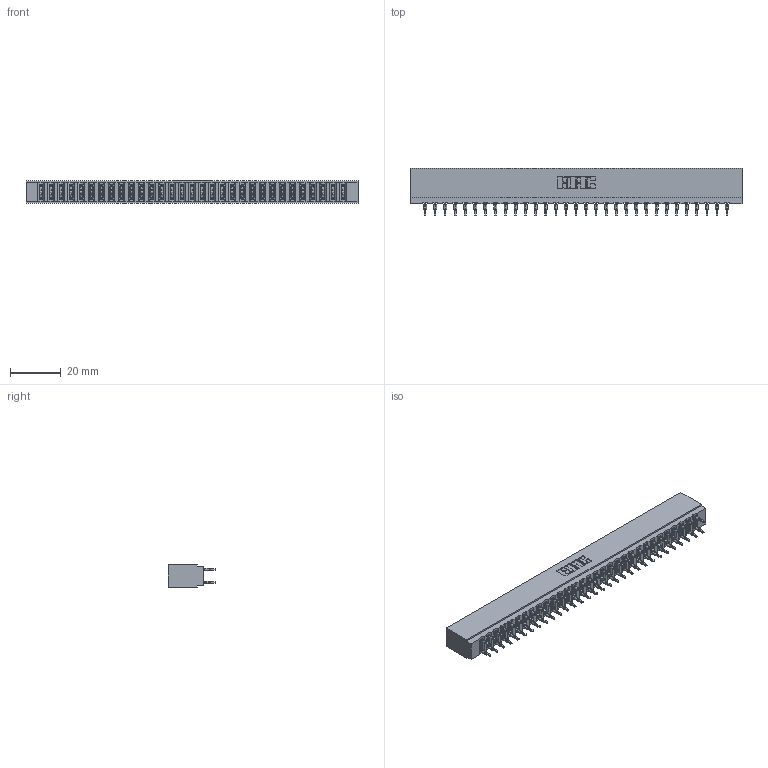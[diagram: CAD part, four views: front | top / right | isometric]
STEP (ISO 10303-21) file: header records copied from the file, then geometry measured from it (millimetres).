
FILE_DESCRIPTION (( 'STEP AP203' ), '1' );
FILE_NAME ('717-062-560-201.STEP', '2026-02-20T18:43:58', ( '' ), ( '' ), 'SwSTEP 2.0', 'SolidWorks 2023', '' );
FILE_SCHEMA (( 'CONFIG_CONTROL_DESIGN' ));
Length unit declared in the file: millimetre
Products named in the file (3): 745-292-001_560; 717-062-560-201; 717 Part_Insulator Option - 06
Assembly tree (63 placements, depth 2):
  717-062-560-201
    717 Part_Insulator Option - 06
    745-292-001_560  x62
Bounding box: 130.71 x 18.78 x 8.89 mm (x, y, z)
Volume: 11600.5 mm3; surface area: 18689 mm2
Topology: 63 solids, 63 shells, 6232 faces, 17053 edges, 10830 vertices
Faces by surface type: plane 3247, cylinder 1373, bspline 1240, torus 372
Entity records: 54968 total; most frequent: CARTESIAN_POINT 10049, ORIENTED_EDGE 9462, DIRECTION 8275, EDGE_CURVE 4731, LINE 4355, VECTOR 4355, VERTEX_POINT 3022, AXIS2_PLACEMENT_3D 1960
